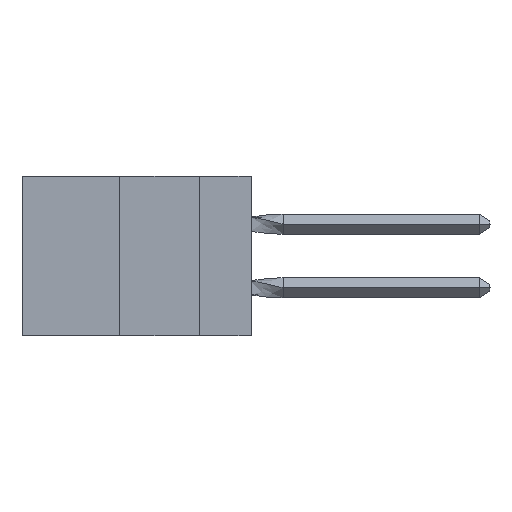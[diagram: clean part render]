
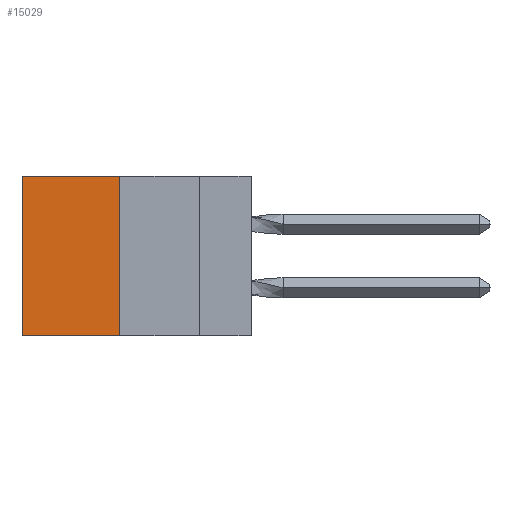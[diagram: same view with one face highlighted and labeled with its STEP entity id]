
A CAD part, left-side view. The second image highlights one B-rep face of the part: STEP entity #15029.
In plain terms, the highlighted planar face has unit normal (-1, 0, 0).
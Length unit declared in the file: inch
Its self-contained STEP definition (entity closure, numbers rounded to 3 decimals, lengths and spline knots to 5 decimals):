
#176 = VECTOR ( 'NONE', #10163, 39.37008 ) ;
#593 = CARTESIAN_POINT ( 'NONE',  ( 0.305, 0.72, 0. ) ) ;
#2696 = FACE_OUTER_BOUND ( 'NONE', #3764, .T. ) ;
#2702 = LINE ( 'NONE', #29561, #18925 ) ;
#3764 = EDGE_LOOP ( 'NONE', ( #9679, #17456, #34973, #20757 ) ) ;
#3871 = EDGE_CURVE ( 'NONE', #22789, #16603, #11091, .T. ) ;
#4431 = EDGE_CURVE ( 'NONE', #22789, #11675, #8747, .T. ) ;
#7920 = CARTESIAN_POINT ( 'NONE',  ( 0.305, 0.413, -0.5 ) ) ;
#8501 = DIRECTION ( 'NONE',  ( 0., 1., 0. ) ) ;
#8747 = LINE ( 'NONE', #34546, #25008 ) ;
#9679 = ORIENTED_EDGE ( 'NONE', *, *, #35119, .T. ) ;
#10163 = DIRECTION ( 'NONE',  ( 0., 0., -1. ) ) ;
#11091 = LINE ( 'NONE', #7920, #37298 ) ;
#11675 = VERTEX_POINT ( 'NONE', #593 ) ;
#12541 = CARTESIAN_POINT ( 'NONE',  ( 0.305, 0.72, -0.5 ) ) ;
#14240 = DIRECTION ( 'NONE',  ( 1., 0., 0. ) ) ;
#14480 = CARTESIAN_POINT ( 'NONE',  ( 0.305, 0.413, -0.5 ) ) ;
#15029 = ADVANCED_FACE ( 'NONE', ( #2696 ), #20040, .F. ) ;
#15594 = CARTESIAN_POINT ( 'NONE',  ( 0.305, 0.72, -0.5 ) ) ;
#16603 = VERTEX_POINT ( 'NONE', #23000 ) ;
#17456 = ORIENTED_EDGE ( 'NONE', *, *, #29710, .F. ) ;
#18925 = VECTOR ( 'NONE', #23501, 39.37008 ) ;
#19131 = VERTEX_POINT ( 'NONE', #12541 ) ;
#20040 = PLANE ( 'NONE',  #28996 ) ;
#20757 = ORIENTED_EDGE ( 'NONE', *, *, #4431, .T. ) ;
#22789 = VERTEX_POINT ( 'NONE', #25564 ) ;
#23000 = CARTESIAN_POINT ( 'NONE',  ( 0.305, 0.413, -0.5 ) ) ;
#23501 = DIRECTION ( 'NONE',  ( 0., 1., 0. ) ) ;
#25008 = VECTOR ( 'NONE', #8501, 39.37008 ) ;
#25564 = CARTESIAN_POINT ( 'NONE',  ( 0.305, 0.413, 0. ) ) ;
#28996 = AXIS2_PLACEMENT_3D ( 'NONE', #14480, #14240, #31943 ) ;
#29561 = CARTESIAN_POINT ( 'NONE',  ( 0.305, 0.413, -0.5 ) ) ;
#29710 = EDGE_CURVE ( 'NONE', #16603, #19131, #2702, .T. ) ;
#31943 = DIRECTION ( 'NONE',  ( 0., 0., -1. ) ) ;
#33716 = DIRECTION ( 'NONE',  ( 0., 0., -1. ) ) ;
#34546 = CARTESIAN_POINT ( 'NONE',  ( 0.305, 0.413, 0. ) ) ;
#34973 = ORIENTED_EDGE ( 'NONE', *, *, #3871, .F. ) ;
#35119 = EDGE_CURVE ( 'NONE', #11675, #19131, #35992, .T. ) ;
#35992 = LINE ( 'NONE', #15594, #176 ) ;
#37298 = VECTOR ( 'NONE', #33716, 39.37008 ) ;
